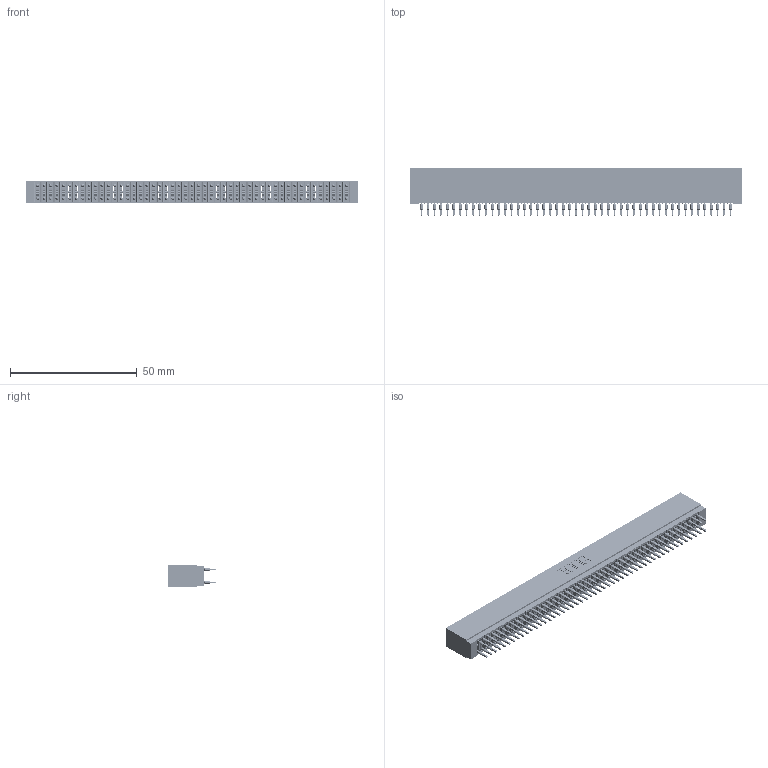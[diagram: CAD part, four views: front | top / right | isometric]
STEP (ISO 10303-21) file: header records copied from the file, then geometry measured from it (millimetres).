
FILE_DESCRIPTION (( 'STEP AP203' ), '1' );
FILE_NAME ('725-098-560-201.STEP', '2026-02-24T19:54:34', ( '' ), ( '' ), 'SwSTEP 2.0', 'SolidWorks 2023', '' );
FILE_SCHEMA (( 'CONFIG_CONTROL_DESIGN' ));
Length unit declared in the file: millimetre
Products named in the file (3): 745-292-001_560; 725-098-560-201; 725 Part_Insulator Option - 01
Assembly tree (99 placements, depth 2):
  725-098-560-201
    725 Part_Insulator Option - 01
    745-292-001_560  x98
Bounding box: 131.06 x 18.8 x 8.89 mm (x, y, z)
Volume: 10720.3 mm3; surface area: 24337.5 mm2
Topology: 99 solids, 99 shells, 9748 faces, 26665 edges, 16926 vertices
Faces by surface type: plane 5053, cylinder 2147, bspline 1960, torus 588
Entity records: 81824 total; most frequent: CARTESIAN_POINT 14693, ORIENTED_EDGE 14142, DIRECTION 12355, EDGE_CURVE 7071, LINE 6587, VECTOR 6587, VERTEX_POINT 4510, AXIS2_PLACEMENT_3D 2884
